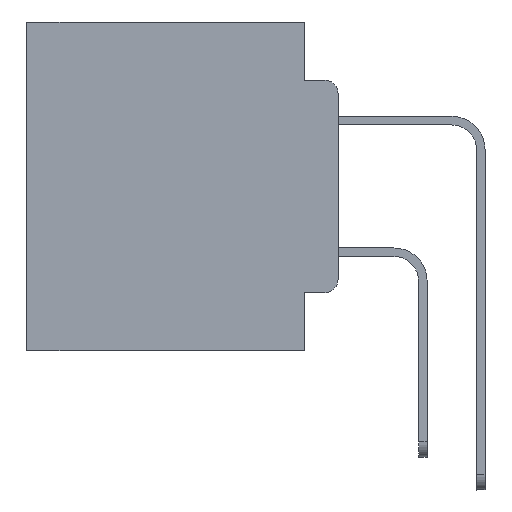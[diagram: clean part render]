
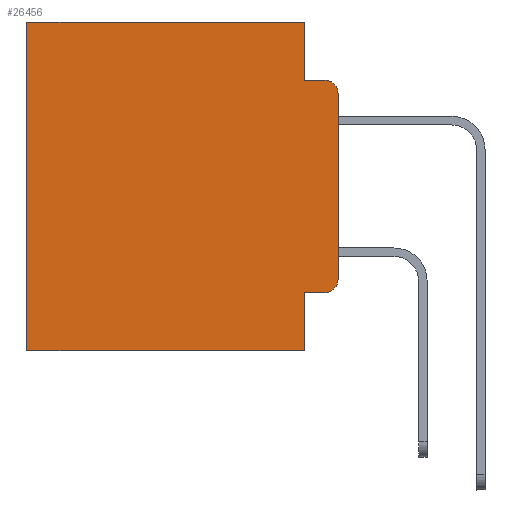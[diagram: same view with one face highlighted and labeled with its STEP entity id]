
A CAD part, left-side view. The second image highlights one B-rep face of the part: STEP entity #26456.
In plain terms, the highlighted planar face has unit normal (-1, 0, 0).
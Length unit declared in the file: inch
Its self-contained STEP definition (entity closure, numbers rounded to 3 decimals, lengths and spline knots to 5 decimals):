
#188 = EDGE_CURVE ( 'NONE', #6481, #23017, #13295, .T. ) ;
#215 = CARTESIAN_POINT ( 'NONE',  ( 0.298, 0., 0. ) ) ;
#307 = VERTEX_POINT ( 'NONE', #4913 ) ;
#412 = CARTESIAN_POINT ( 'NONE',  ( 0.298, 0., 0. ) ) ;
#476 = LINE ( 'NONE', #13532, #17277 ) ;
#495 = CARTESIAN_POINT ( 'NONE',  ( 0.298, 0.02, -0.0885 ) ) ;
#754 = VERTEX_POINT ( 'NONE', #3401 ) ;
#1571 = VERTEX_POINT ( 'NONE', #21154 ) ;
#2267 = CARTESIAN_POINT ( 'NONE',  ( 0.298, 0.473, 0. ) ) ;
#2311 = CARTESIAN_POINT ( 'NONE',  ( 0.298, 0.473, 0. ) ) ;
#3401 = CARTESIAN_POINT ( 'NONE',  ( 0.298, 0.051, -0.4115 ) ) ;
#3579 = LINE ( 'NONE', #16966, #4267 ) ;
#3619 = EDGE_CURVE ( 'NONE', #7214, #15788, #9677, .T. ) ;
#3838 = VECTOR ( 'NONE', #7422, 39.37008 ) ;
#4151 = VECTOR ( 'NONE', #17917, 39.37008 ) ;
#4267 = VECTOR ( 'NONE', #19120, 39.37008 ) ;
#4412 = ORIENTED_EDGE ( 'NONE', *, *, #10382, .F. ) ;
#4913 = CARTESIAN_POINT ( 'NONE',  ( 0.298, 0.051, -0.5 ) ) ;
#5282 = CARTESIAN_POINT ( 'NONE',  ( 0.298, 0.02, -0.3915 ) ) ;
#5371 = EDGE_CURVE ( 'NONE', #1571, #7214, #21768, .T. ) ;
#5824 = EDGE_CURVE ( 'NONE', #307, #23017, #22868, .T. ) ;
#5831 = CARTESIAN_POINT ( 'NONE',  ( 0.298, 0.02, -0.1085 ) ) ;
#5907 = EDGE_CURVE ( 'NONE', #1571, #6481, #15824, .T. ) ;
#6409 = DIRECTION ( 'NONE',  ( 0., -1., 0. ) ) ;
#6481 = VERTEX_POINT ( 'NONE', #2311 ) ;
#6493 = ORIENTED_EDGE ( 'NONE', *, *, #188, .T. ) ;
#6882 = DIRECTION ( 'NONE',  ( 0., 0., -1. ) ) ;
#7214 = VERTEX_POINT ( 'NONE', #18426 ) ;
#7338 = CARTESIAN_POINT ( 'NONE',  ( 0.298, 0.02, -0.4115 ) ) ;
#7422 = DIRECTION ( 'NONE',  ( 0., -1., 0. ) ) ;
#7497 = DIRECTION ( 'NONE',  ( 0., 0., -1. ) ) ;
#7554 = EDGE_CURVE ( 'NONE', #754, #21826, #19451, .T. ) ;
#7585 = CARTESIAN_POINT ( 'NONE',  ( 0.298, 0.051, -0.0885 ) ) ;
#7653 = VERTEX_POINT ( 'NONE', #24416 ) ;
#7761 = EDGE_CURVE ( 'NONE', #12838, #15788, #14077, .T. ) ;
#7899 = VECTOR ( 'NONE', #6409, 39.37008 ) ;
#8053 = DIRECTION ( 'NONE',  ( 0., 0., -1. ) ) ;
#9677 = LINE ( 'NONE', #7585, #3838 ) ;
#10382 = EDGE_CURVE ( 'NONE', #754, #307, #3579, .T. ) ;
#10665 = DIRECTION ( 'NONE',  ( 0., 0., -1. ) ) ;
#11671 = ORIENTED_EDGE ( 'NONE', *, *, #7554, .T. ) ;
#12838 = VERTEX_POINT ( 'NONE', #15057 ) ;
#13029 = ORIENTED_EDGE ( 'NONE', *, *, #5824, .F. ) ;
#13295 = LINE ( 'NONE', #2267, #23371 ) ;
#13532 = CARTESIAN_POINT ( 'NONE',  ( 0.298, 0., 0. ) ) ;
#14022 = DIRECTION ( 'NONE',  ( 0., 0., -1. ) ) ;
#14077 = CIRCLE ( 'NONE', #20068, 0.02 ) ;
#14417 = ORIENTED_EDGE ( 'NONE', *, *, #5371, .F. ) ;
#15057 = CARTESIAN_POINT ( 'NONE',  ( 0.298, 0., -0.1085 ) ) ;
#15701 = DIRECTION ( 'NONE',  ( 0., 0., -1. ) ) ;
#15788 = VERTEX_POINT ( 'NONE', #495 ) ;
#15824 = LINE ( 'NONE', #412, #4151 ) ;
#16966 = CARTESIAN_POINT ( 'NONE',  ( 0.298, 0.051, 0. ) ) ;
#17160 = VECTOR ( 'NONE', #26281, 39.37008 ) ;
#17277 = VECTOR ( 'NONE', #15701, 39.37008 ) ;
#17735 = PLANE ( 'NONE',  #25623 ) ;
#17917 = DIRECTION ( 'NONE',  ( 0., 1., 0. ) ) ;
#18426 = CARTESIAN_POINT ( 'NONE',  ( 0.298, 0.051, -0.0885 ) ) ;
#19120 = DIRECTION ( 'NONE',  ( 0., 0., -1. ) ) ;
#19211 = EDGE_CURVE ( 'NONE', #12838, #7653, #476, .T. ) ;
#19451 = LINE ( 'NONE', #25914, #7899 ) ;
#19789 = ORIENTED_EDGE ( 'NONE', *, *, #25007, .T. ) ;
#19805 = CARTESIAN_POINT ( 'NONE',  ( 0.298, 0., -0.5 ) ) ;
#19894 = DIRECTION ( 'NONE',  ( 1., 0., 0. ) ) ;
#20068 = AXIS2_PLACEMENT_3D ( 'NONE', #5831, #21021, #8053 ) ;
#20496 = DIRECTION ( 'NONE',  ( -1., 0., 0. ) ) ;
#21021 = DIRECTION ( 'NONE',  ( -1., 0., 0. ) ) ;
#21091 = VECTOR ( 'NONE', #14022, 39.37008 ) ;
#21154 = CARTESIAN_POINT ( 'NONE',  ( 0.298, 0.051, 0. ) ) ;
#21500 = CIRCLE ( 'NONE', #23956, 0.02 ) ;
#21768 = LINE ( 'NONE', #26881, #21091 ) ;
#21826 = VERTEX_POINT ( 'NONE', #7338 ) ;
#22868 = LINE ( 'NONE', #19805, #17160 ) ;
#23017 = VERTEX_POINT ( 'NONE', #24345 ) ;
#23371 = VECTOR ( 'NONE', #10665, 39.37008 ) ;
#23747 = FACE_OUTER_BOUND ( 'NONE', #27377, .T. ) ;
#23956 = AXIS2_PLACEMENT_3D ( 'NONE', #5282, #20496, #7497 ) ;
#24345 = CARTESIAN_POINT ( 'NONE',  ( 0.298, 0.473, -0.5 ) ) ;
#24416 = CARTESIAN_POINT ( 'NONE',  ( 0.298, 0., -0.3915 ) ) ;
#24462 = ORIENTED_EDGE ( 'NONE', *, *, #5907, .T. ) ;
#25007 = EDGE_CURVE ( 'NONE', #21826, #7653, #21500, .T. ) ;
#25471 = ORIENTED_EDGE ( 'NONE', *, *, #19211, .F. ) ;
#25623 = AXIS2_PLACEMENT_3D ( 'NONE', #215, #19894, #6882 ) ;
#25914 = CARTESIAN_POINT ( 'NONE',  ( 0.298, 0.051, -0.4115 ) ) ;
#26281 = DIRECTION ( 'NONE',  ( 0., 1., 0. ) ) ;
#26456 = ADVANCED_FACE ( 'NONE', ( #23747 ), #17735, .F. ) ;
#26569 = ORIENTED_EDGE ( 'NONE', *, *, #7761, .T. ) ;
#26813 = ORIENTED_EDGE ( 'NONE', *, *, #3619, .F. ) ;
#26881 = CARTESIAN_POINT ( 'NONE',  ( 0.298, 0.051, 0. ) ) ;
#27377 = EDGE_LOOP ( 'NONE', ( #25471, #26569, #26813, #14417, #24462, #6493, #13029, #4412, #11671, #19789 ) ) ;
